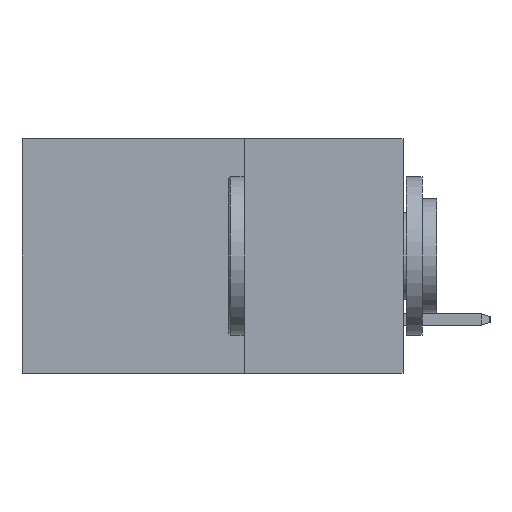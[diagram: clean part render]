
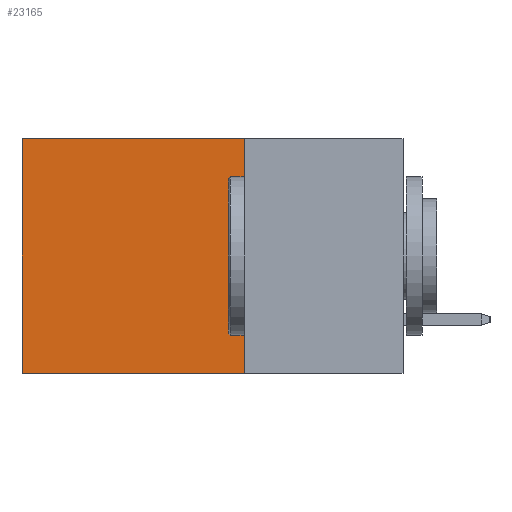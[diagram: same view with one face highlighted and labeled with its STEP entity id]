
A CAD part, left-side view. The second image highlights one B-rep face of the part: STEP entity #23165.
In plain terms, the highlighted planar face has unit normal (-1, 0, 0).
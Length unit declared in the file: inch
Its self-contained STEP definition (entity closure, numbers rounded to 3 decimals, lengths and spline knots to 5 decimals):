
#654 = VERTEX_POINT ( 'NONE', #20697 ) ;
#777 = EDGE_CURVE ( 'NONE', #5299, #19150, #1468, .T. ) ;
#1393 = LINE ( 'NONE', #1523, #21111 ) ;
#1468 = LINE ( 'NONE', #23584, #21147 ) ;
#1522 = VERTEX_POINT ( 'NONE', #24780 ) ;
#1523 = CARTESIAN_POINT ( 'NONE',  ( 0.2875, 0.25, -0.37 ) ) ;
#2521 = CARTESIAN_POINT ( 'NONE',  ( 0.2875, 0.25, 0. ) ) ;
#3457 = DIRECTION ( 'NONE',  ( 0., 0., -1. ) ) ;
#4107 = DIRECTION ( 'NONE',  ( 0., 1., 0. ) ) ;
#4127 = EDGE_LOOP ( 'NONE', ( #19361, #16020, #12626, #22801 ) ) ;
#5299 = VERTEX_POINT ( 'NONE', #19844 ) ;
#6288 = EDGE_CURVE ( 'NONE', #1522, #19150, #1393, .T. ) ;
#6354 = PLANE ( 'NONE',  #9798 ) ;
#7382 = EDGE_CURVE ( 'NONE', #654, #5299, #11780, .T. ) ;
#9798 = AXIS2_PLACEMENT_3D ( 'NONE', #2521, #10595, #18690 ) ;
#10503 = CARTESIAN_POINT ( 'NONE',  ( 0.2875, 0.6, -0.37 ) ) ;
#10595 = DIRECTION ( 'NONE',  ( 1., 0., 0. ) ) ;
#11780 = LINE ( 'NONE', #25816, #24109 ) ;
#12626 = ORIENTED_EDGE ( 'NONE', *, *, #24964, .F. ) ;
#12720 = FACE_OUTER_BOUND ( 'NONE', #4127, .T. ) ;
#15083 = CARTESIAN_POINT ( 'NONE',  ( 0.2875, 0.25, 0. ) ) ;
#16020 = ORIENTED_EDGE ( 'NONE', *, *, #6288, .F. ) ;
#16245 = VECTOR ( 'NONE', #23133, 39.37008 ) ;
#18690 = DIRECTION ( 'NONE',  ( 0., 0., -1. ) ) ;
#19150 = VERTEX_POINT ( 'NONE', #10503 ) ;
#19361 = ORIENTED_EDGE ( 'NONE', *, *, #777, .T. ) ;
#19844 = CARTESIAN_POINT ( 'NONE',  ( 0.2875, 0.6, 0. ) ) ;
#20697 = CARTESIAN_POINT ( 'NONE',  ( 0.2875, 0.25, 0. ) ) ;
#21111 = VECTOR ( 'NONE', #21528, 39.37008 ) ;
#21147 = VECTOR ( 'NONE', #3457, 39.37008 ) ;
#21528 = DIRECTION ( 'NONE',  ( 0., 1., 0. ) ) ;
#21555 = LINE ( 'NONE', #15083, #16245 ) ;
#22801 = ORIENTED_EDGE ( 'NONE', *, *, #7382, .T. ) ;
#23133 = DIRECTION ( 'NONE',  ( 0., 0., -1. ) ) ;
#23165 = ADVANCED_FACE ( 'NONE', ( #12720 ), #6354, .F. ) ;
#23584 = CARTESIAN_POINT ( 'NONE',  ( 0.2875, 0.6, 0. ) ) ;
#24109 = VECTOR ( 'NONE', #4107, 39.37008 ) ;
#24780 = CARTESIAN_POINT ( 'NONE',  ( 0.2875, 0.25, -0.37 ) ) ;
#24964 = EDGE_CURVE ( 'NONE', #654, #1522, #21555, .T. ) ;
#25816 = CARTESIAN_POINT ( 'NONE',  ( 0.2875, 0.25, 0. ) ) ;
